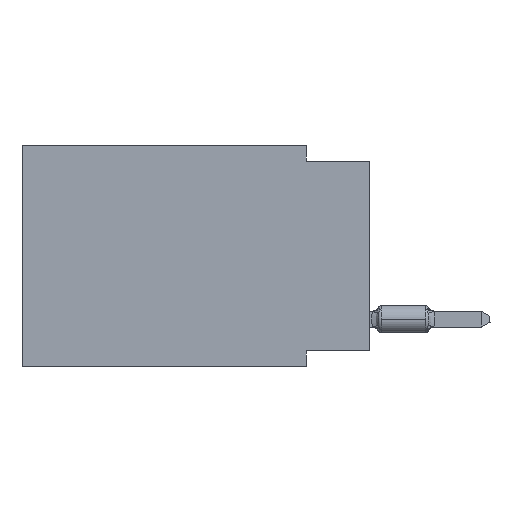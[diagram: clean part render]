
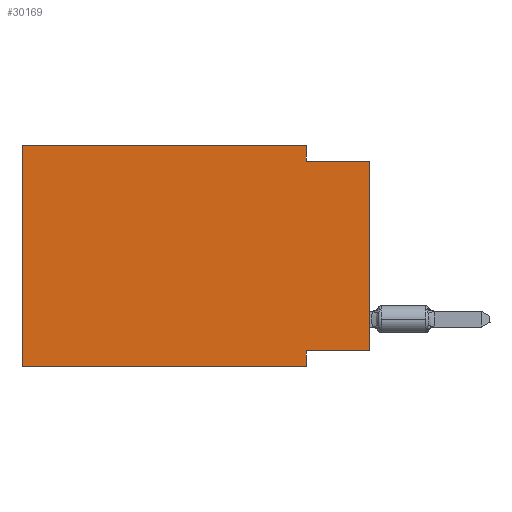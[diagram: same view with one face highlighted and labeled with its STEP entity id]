
A CAD part, left-side view. The second image highlights one B-rep face of the part: STEP entity #30169.
In plain terms, the highlighted planar face has unit normal (-1, 0, 0).
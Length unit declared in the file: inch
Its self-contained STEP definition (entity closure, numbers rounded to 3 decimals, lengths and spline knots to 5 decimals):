
#68 = EDGE_LOOP ( 'NONE', ( #814, #4625, #41655, #2232, #51447, #44358, #46172, #13480 ) ) ;
#814 = ORIENTED_EDGE ( 'NONE', *, *, #49087, .T. ) ;
#2232 = ORIENTED_EDGE ( 'NONE', *, *, #10955, .F. ) ;
#2494 = DIRECTION ( 'NONE',  ( 0., -1., 0. ) ) ;
#3067 = VERTEX_POINT ( 'NONE', #10001 ) ;
#4380 = LINE ( 'NONE', #33991, #31765 ) ;
#4625 = ORIENTED_EDGE ( 'NONE', *, *, #31478, .F. ) ;
#5804 = DIRECTION ( 'NONE',  ( 0., 0., 1. ) ) ;
#6726 = PLANE ( 'NONE',  #7350 ) ;
#7350 = AXIS2_PLACEMENT_3D ( 'NONE', #14946, #52223, #51959 ) ;
#7749 = EDGE_CURVE ( 'NONE', #14275, #35371, #37367, .T. ) ;
#10001 = CARTESIAN_POINT ( 'NONE',  ( 0., 0., -0.025 ) ) ;
#10012 = LINE ( 'NONE', #34972, #46757 ) ;
#10603 = VERTEX_POINT ( 'NONE', #27793 ) ;
#10955 = EDGE_CURVE ( 'NONE', #44875, #14275, #35942, .T. ) ;
#11324 = CARTESIAN_POINT ( 'NONE',  ( 0., 0.55, -0.35 ) ) ;
#12852 = CARTESIAN_POINT ( 'NONE',  ( 0., 0.1, -0.325 ) ) ;
#13480 = ORIENTED_EDGE ( 'NONE', *, *, #30218, .F. ) ;
#14055 = CARTESIAN_POINT ( 'NONE',  ( 0., 0., -0.325 ) ) ;
#14275 = VERTEX_POINT ( 'NONE', #32031 ) ;
#14277 = VECTOR ( 'NONE', #35675, 39.37008 ) ;
#14946 = CARTESIAN_POINT ( 'NONE',  ( 0., 0.55, 0. ) ) ;
#17951 = VECTOR ( 'NONE', #28077, 39.37008 ) ;
#18532 = LINE ( 'NONE', #31681, #30174 ) ;
#18752 = VECTOR ( 'NONE', #5804, 39.37008 ) ;
#18951 = CARTESIAN_POINT ( 'NONE',  ( 0., 0., 0. ) ) ;
#19572 = VERTEX_POINT ( 'NONE', #12852 ) ;
#20934 = VERTEX_POINT ( 'NONE', #22010 ) ;
#22010 = CARTESIAN_POINT ( 'NONE',  ( 0., 0.1, -0.35 ) ) ;
#22636 = DIRECTION ( 'NONE',  ( 0., 1., 0. ) ) ;
#23619 = CARTESIAN_POINT ( 'NONE',  ( 0., 0.55, 0. ) ) ;
#23706 = FACE_OUTER_BOUND ( 'NONE', #68, .T. ) ;
#27793 = CARTESIAN_POINT ( 'NONE',  ( 0., 0.55, -0.35 ) ) ;
#28077 = DIRECTION ( 'NONE',  ( 0., -1., 0. ) ) ;
#28619 = VECTOR ( 'NONE', #2494, 39.37008 ) ;
#28878 = VERTEX_POINT ( 'NONE', #14055 ) ;
#29082 = DIRECTION ( 'NONE',  ( 0., 0., -1. ) ) ;
#30169 = ADVANCED_FACE ( 'NONE', ( #23706 ), #6726, .F. ) ;
#30174 = VECTOR ( 'NONE', #51965, 39.37008 ) ;
#30218 = EDGE_CURVE ( 'NONE', #28878, #19572, #10012, .T. ) ;
#31478 = EDGE_CURVE ( 'NONE', #35371, #3067, #18532, .T. ) ;
#31681 = CARTESIAN_POINT ( 'NONE',  ( 0., 0., -0.025 ) ) ;
#31765 = VECTOR ( 'NONE', #29082, 39.37008 ) ;
#32031 = CARTESIAN_POINT ( 'NONE',  ( 0., 0.1, 0. ) ) ;
#32719 = CARTESIAN_POINT ( 'NONE',  ( 0., 0.1, -0.025 ) ) ;
#33254 = CARTESIAN_POINT ( 'NONE',  ( 0., 0.1, 0. ) ) ;
#33991 = CARTESIAN_POINT ( 'NONE',  ( 0., 0.1, -0.35 ) ) ;
#34972 = CARTESIAN_POINT ( 'NONE',  ( 0., 0., -0.325 ) ) ;
#35371 = VERTEX_POINT ( 'NONE', #32719 ) ;
#35675 = DIRECTION ( 'NONE',  ( 0., 0., 1. ) ) ;
#35942 = LINE ( 'NONE', #39243, #28619 ) ;
#36813 = DIRECTION ( 'NONE',  ( 0., 0., -1. ) ) ;
#37367 = LINE ( 'NONE', #33254, #53534 ) ;
#39243 = CARTESIAN_POINT ( 'NONE',  ( 0., 0.55, 0. ) ) ;
#41655 = ORIENTED_EDGE ( 'NONE', *, *, #7749, .F. ) ;
#43094 = CARTESIAN_POINT ( 'NONE',  ( 0., 0.55, 0. ) ) ;
#43902 = LINE ( 'NONE', #18951, #14277 ) ;
#44358 = ORIENTED_EDGE ( 'NONE', *, *, #52856, .T. ) ;
#44875 = VERTEX_POINT ( 'NONE', #23619 ) ;
#46172 = ORIENTED_EDGE ( 'NONE', *, *, #50400, .F. ) ;
#46757 = VECTOR ( 'NONE', #22636, 39.37008 ) ;
#48884 = EDGE_CURVE ( 'NONE', #10603, #44875, #51561, .T. ) ;
#49087 = EDGE_CURVE ( 'NONE', #28878, #3067, #43902, .T. ) ;
#50400 = EDGE_CURVE ( 'NONE', #19572, #20934, #4380, .T. ) ;
#51447 = ORIENTED_EDGE ( 'NONE', *, *, #48884, .F. ) ;
#51561 = LINE ( 'NONE', #43094, #18752 ) ;
#51959 = DIRECTION ( 'NONE',  ( 0., 0., -1. ) ) ;
#51965 = DIRECTION ( 'NONE',  ( 0., -1., 0. ) ) ;
#52223 = DIRECTION ( 'NONE',  ( 1., 0., 0. ) ) ;
#52729 = LINE ( 'NONE', #11324, #17951 ) ;
#52856 = EDGE_CURVE ( 'NONE', #10603, #20934, #52729, .T. ) ;
#53534 = VECTOR ( 'NONE', #36813, 39.37008 ) ;
